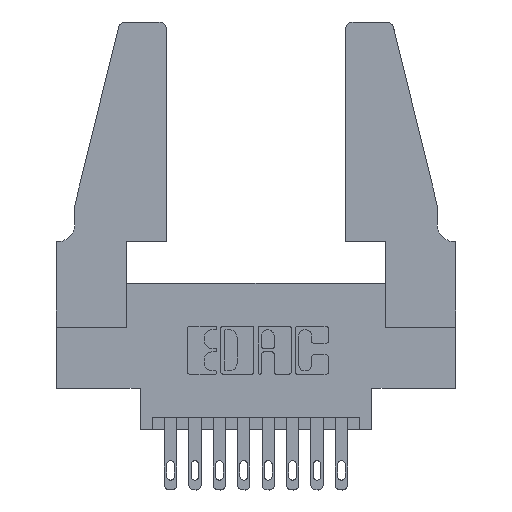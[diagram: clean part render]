
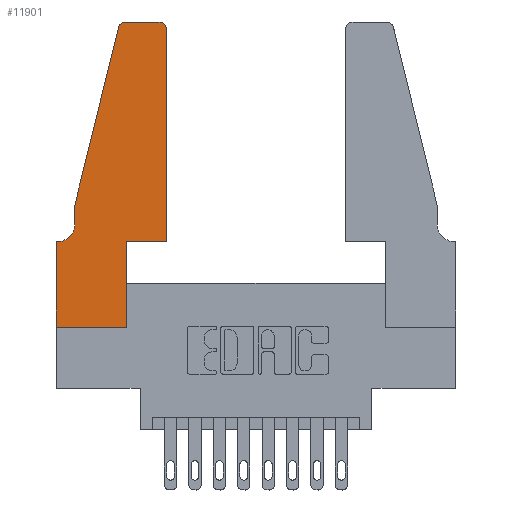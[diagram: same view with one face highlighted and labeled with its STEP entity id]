
A CAD part, top view. The second image highlights one B-rep face of the part: STEP entity #11901.
In plain terms, the highlighted planar face has unit normal (0, 0, 1).
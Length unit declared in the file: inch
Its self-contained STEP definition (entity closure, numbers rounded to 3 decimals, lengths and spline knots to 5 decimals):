
#65 = DIRECTION ( 'NONE',  ( 0., 0., 1. ) ) ;
#72 = VERTEX_POINT ( 'NONE', #8395 ) ;
#200 = VECTOR ( 'NONE', #11649, 39.37008 ) ;
#338 = VECTOR ( 'NONE', #12254, 39.37008 ) ;
#620 = VECTOR ( 'NONE', #10264, 39.37008 ) ;
#646 = ORIENTED_EDGE ( 'NONE', *, *, #3050, .T. ) ;
#927 = CARTESIAN_POINT ( 'NONE',  ( 0., 0., 0.37 ) ) ;
#990 = AXIS2_PLACEMENT_3D ( 'NONE', #7893, #5830, #1801 ) ;
#1076 = AXIS2_PLACEMENT_3D ( 'NONE', #8579, #1478, #10555 ) ;
#1085 = CARTESIAN_POINT ( 'NONE',  ( 0.0755, 0.5, 0.37 ) ) ;
#1111 = DIRECTION ( 'NONE',  ( -1., 0., 0. ) ) ;
#1175 = VECTOR ( 'NONE', #7400, 39.37008 ) ;
#1478 = DIRECTION ( 'NONE',  ( 0., 0., -1. ) ) ;
#1497 = LINE ( 'NONE', #6103, #1811 ) ;
#1801 = DIRECTION ( 'NONE',  ( 1., 0., 0. ) ) ;
#1811 = VECTOR ( 'NONE', #1111, 39.37008 ) ;
#1816 = CARTESIAN_POINT ( 'NONE',  ( 0., 0., 0.37 ) ) ;
#1910 = CARTESIAN_POINT ( 'NONE',  ( 0.0055, 0.35, 0.37 ) ) ;
#2015 = CARTESIAN_POINT ( 'NONE',  ( 0.0755, 0.5, 0.37 ) ) ;
#2022 = LINE ( 'NONE', #8189, #620 ) ;
#2228 = LINE ( 'NONE', #1816, #3782 ) ;
#2249 = LINE ( 'NONE', #5568, #200 ) ;
#2618 = VERTEX_POINT ( 'NONE', #3384 ) ;
#2872 = EDGE_CURVE ( 'NONE', #8966, #7697, #2022, .T. ) ;
#2934 = CARTESIAN_POINT ( 'NONE',  ( 0.2865, 0.35, 0.37 ) ) ;
#3033 = CIRCLE ( 'NONE', #1076, 0.07 ) ;
#3037 = ORIENTED_EDGE ( 'NONE', *, *, #3545, .T. ) ;
#3050 = EDGE_CURVE ( 'NONE', #7687, #72, #11822, .T. ) ;
#3322 = VECTOR ( 'NONE', #4390, 39.37008 ) ;
#3332 = ORIENTED_EDGE ( 'NONE', *, *, #12115, .T. ) ;
#3384 = CARTESIAN_POINT ( 'NONE',  ( 0.2865, 0., 0.37 ) ) ;
#3426 = ORIENTED_EDGE ( 'NONE', *, *, #4368, .T. ) ;
#3545 = EDGE_CURVE ( 'NONE', #7697, #8036, #11805, .T. ) ;
#3552 = VECTOR ( 'NONE', #8501, 39.37008 ) ;
#3699 = VERTEX_POINT ( 'NONE', #10373 ) ;
#3749 = CARTESIAN_POINT ( 'NONE',  ( 0.4505, 1.22, 0.37 ) ) ;
#3782 = VECTOR ( 'NONE', #6032, 39.37008 ) ;
#4096 = CARTESIAN_POINT ( 'NONE',  ( 0.4505, 0.35, 0.37 ) ) ;
#4368 = EDGE_CURVE ( 'NONE', #8036, #7687, #7263, .T. ) ;
#4376 = CARTESIAN_POINT ( 'NONE',  ( 0.284, 1.22, 0.37 ) ) ;
#4390 = DIRECTION ( 'NONE',  ( 0., -1., 0. ) ) ;
#4444 = VECTOR ( 'NONE', #10997, 39.37008 ) ;
#4832 = VERTEX_POINT ( 'NONE', #13013 ) ;
#5568 = CARTESIAN_POINT ( 'NONE',  ( 0.4505, 0.35, 0.37 ) ) ;
#5695 = PLANE ( 'NONE',  #990 ) ;
#5830 = DIRECTION ( 'NONE',  ( 0., 0., 1. ) ) ;
#5900 = ORIENTED_EDGE ( 'NONE', *, *, #10906, .T. ) ;
#6032 = DIRECTION ( 'NONE',  ( 1., 0., 0. ) ) ;
#6103 = CARTESIAN_POINT ( 'NONE',  ( 0.0755, 0.35, 0.37 ) ) ;
#6338 = DIRECTION ( 'NONE',  ( 0., 0., 1. ) ) ;
#6361 = FACE_OUTER_BOUND ( 'NONE', #12479, .T. ) ;
#6447 = AXIS2_PLACEMENT_3D ( 'NONE', #9026, #65, #11085 ) ;
#6530 = LINE ( 'NONE', #1085, #338 ) ;
#6605 = AXIS2_PLACEMENT_3D ( 'NONE', #4376, #6338, #9310 ) ;
#6714 = EDGE_CURVE ( 'NONE', #4832, #8966, #2249, .T. ) ;
#7263 = LINE ( 'NONE', #10460, #3552 ) ;
#7360 = LINE ( 'NONE', #2015, #1175 ) ;
#7400 = DIRECTION ( 'NONE',  ( -0.239, -0.971, 0. ) ) ;
#7523 = LINE ( 'NONE', #2934, #4444 ) ;
#7687 = VERTEX_POINT ( 'NONE', #9312 ) ;
#7697 = VERTEX_POINT ( 'NONE', #3749 ) ;
#7893 = CARTESIAN_POINT ( 'NONE',  ( 0., 0.35, 0.37 ) ) ;
#8036 = VERTEX_POINT ( 'NONE', #13083 ) ;
#8189 = CARTESIAN_POINT ( 'NONE',  ( 0.4505, 0.35, 0.37 ) ) ;
#8368 = ORIENTED_EDGE ( 'NONE', *, *, #10168, .T. ) ;
#8395 = CARTESIAN_POINT ( 'NONE',  ( 0.25487, 1.22718, 0.37 ) ) ;
#8501 = DIRECTION ( 'NONE',  ( -1., 0., 0. ) ) ;
#8579 = CARTESIAN_POINT ( 'NONE',  ( 0.0055, 0.42, 0.37 ) ) ;
#8966 = VERTEX_POINT ( 'NONE', #4096 ) ;
#9026 = CARTESIAN_POINT ( 'NONE',  ( 0.4205, 1.22, 0.37 ) ) ;
#9256 = VERTEX_POINT ( 'NONE', #1910 ) ;
#9310 = DIRECTION ( 'NONE',  ( 1., 0., 0. ) ) ;
#9312 = CARTESIAN_POINT ( 'NONE',  ( 0.284, 1.25, 0.37 ) ) ;
#9738 = CARTESIAN_POINT ( 'NONE',  ( 0.0755, 0.42, 0.37 ) ) ;
#9995 = ORIENTED_EDGE ( 'NONE', *, *, #11163, .T. ) ;
#10168 = EDGE_CURVE ( 'NONE', #9256, #10915, #1497, .T. ) ;
#10264 = DIRECTION ( 'NONE',  ( 0., 1., 0. ) ) ;
#10373 = CARTESIAN_POINT ( 'NONE',  ( 0.0755, 0.5, 0.37 ) ) ;
#10460 = CARTESIAN_POINT ( 'NONE',  ( 0.2605, 1.25, 0.37 ) ) ;
#10553 = CARTESIAN_POINT ( 'NONE',  ( 0., 0., 0.37 ) ) ;
#10555 = DIRECTION ( 'NONE',  ( -1., 0., 0. ) ) ;
#10593 = EDGE_CURVE ( 'NONE', #12309, #9256, #3033, .T. ) ;
#10640 = EDGE_CURVE ( 'NONE', #2618, #4832, #7523, .T. ) ;
#10673 = ORIENTED_EDGE ( 'NONE', *, *, #11779, .T. ) ;
#10906 = EDGE_CURVE ( 'NONE', #72, #3699, #7360, .T. ) ;
#10915 = VERTEX_POINT ( 'NONE', #11354 ) ;
#10963 = ORIENTED_EDGE ( 'NONE', *, *, #2872, .T. ) ;
#10997 = DIRECTION ( 'NONE',  ( 0., 1., 0. ) ) ;
#11085 = DIRECTION ( 'NONE',  ( 1., 0., 0. ) ) ;
#11163 = EDGE_CURVE ( 'NONE', #10915, #12731, #11397, .T. ) ;
#11236 = ORIENTED_EDGE ( 'NONE', *, *, #10593, .T. ) ;
#11354 = CARTESIAN_POINT ( 'NONE',  ( 0., 0.35, 0.37 ) ) ;
#11397 = LINE ( 'NONE', #10553, #3322 ) ;
#11637 = ORIENTED_EDGE ( 'NONE', *, *, #6714, .T. ) ;
#11649 = DIRECTION ( 'NONE',  ( 1., 0., 0. ) ) ;
#11779 = EDGE_CURVE ( 'NONE', #3699, #12309, #6530, .T. ) ;
#11805 = CIRCLE ( 'NONE', #6447, 0.03 ) ;
#11822 = CIRCLE ( 'NONE', #6605, 0.03 ) ;
#11901 = ADVANCED_FACE ( 'NONE', ( #6361 ), #5695, .T. ) ;
#12115 = EDGE_CURVE ( 'NONE', #12731, #2618, #2228, .T. ) ;
#12233 = ORIENTED_EDGE ( 'NONE', *, *, #10640, .T. ) ;
#12254 = DIRECTION ( 'NONE',  ( 0., -1., 0. ) ) ;
#12309 = VERTEX_POINT ( 'NONE', #9738 ) ;
#12479 = EDGE_LOOP ( 'NONE', ( #3426, #646, #5900, #10673, #11236, #8368, #9995, #3332, #12233, #11637, #10963, #3037 ) ) ;
#12731 = VERTEX_POINT ( 'NONE', #927 ) ;
#13013 = CARTESIAN_POINT ( 'NONE',  ( 0.2865, 0.35, 0.37 ) ) ;
#13083 = CARTESIAN_POINT ( 'NONE',  ( 0.4205, 1.25, 0.37 ) ) ;
